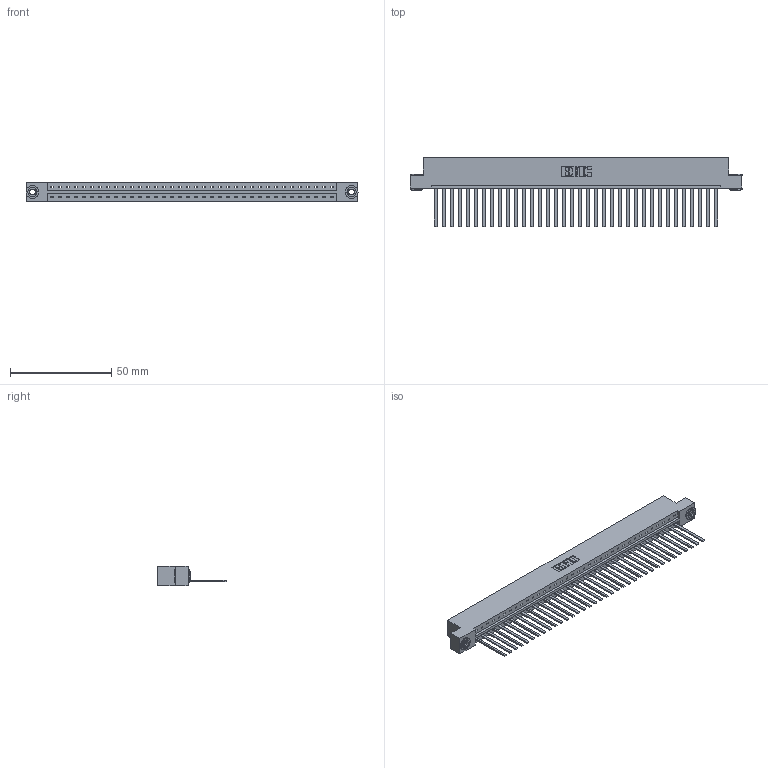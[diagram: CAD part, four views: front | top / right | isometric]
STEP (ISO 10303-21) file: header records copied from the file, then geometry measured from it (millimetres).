
FILE_DESCRIPTION (( 'STEP AP203' ), '1' );
FILE_NAME ('833-036-544-103.STEP', '2020-06-03T03:23:07', ( '' ), ( '' ), 'SwSTEP 2.0', 'SolidWorks 2020', '' );
FILE_SCHEMA (( 'CONFIG_CONTROL_DESIGN' ));
Length unit declared in the file: inch
Products named in the file (4): 833 Part_Flush - .156 Dia - TH; 833-036-544-103; 345-250-002_345-250-002-102; 345-292-001_345-293-144
Assembly tree (39 placements, depth 2):
  833-036-544-103
    833 Part_Flush - .156 Dia - TH
    345-292-001_345-293-144  x36
    345-250-002_345-250-002-102  x2
Bounding box: 164.19 x 34.3 x 9.4 mm (x, y, z)
Volume: 16906.4 mm3; surface area: 19836.5 mm2
Topology: 39 solids, 39 shells, 2024 faces, 6075 edges, 3998 vertices
Faces by surface type: plane 1448, cylinder 568, cone 8
Entity records: 23250 total; most frequent: CARTESIAN_POINT 3989, ORIENTED_EDGE 3954, DIRECTION 3407, EDGE_CURVE 1977, LINE 1829, VECTOR 1829, VERTEX_POINT 1314, AXIS2_PLACEMENT_3D 789
